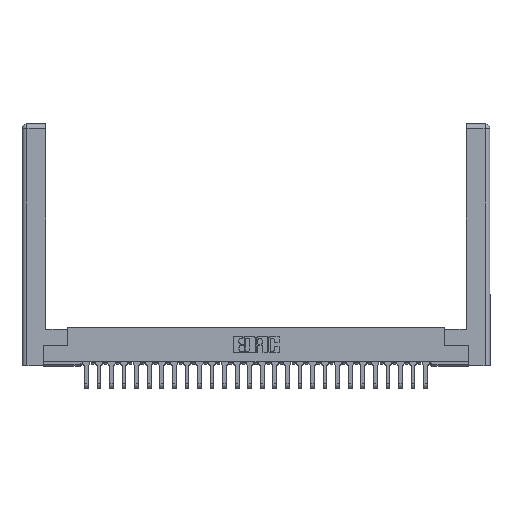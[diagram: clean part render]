
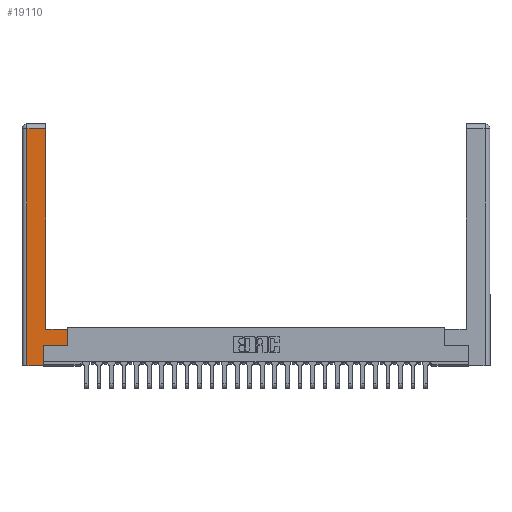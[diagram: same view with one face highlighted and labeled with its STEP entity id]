
A CAD part, top view. The second image highlights one B-rep face of the part: STEP entity #19110.
In plain terms, the highlighted planar face has unit normal (0, 0, 1).
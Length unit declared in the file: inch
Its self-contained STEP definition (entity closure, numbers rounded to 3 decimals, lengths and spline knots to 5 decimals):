
#45 = VECTOR ( 'NONE', #21171, 39.37008 ) ;
#301 = ORIENTED_EDGE ( 'NONE', *, *, #15538, .T. ) ;
#724 = VECTOR ( 'NONE', #25963, 39.37008 ) ;
#1144 = DIRECTION ( 'NONE',  ( 0., 1., 0. ) ) ;
#1430 = LINE ( 'NONE', #19168, #45 ) ;
#1854 = CARTESIAN_POINT ( 'NONE',  ( 0., 0., 0. ) ) ;
#1991 = EDGE_CURVE ( 'NONE', #27890, #3906, #9486, .T. ) ;
#2166 = CARTESIAN_POINT ( 'NONE',  ( 0.265, 0., 0. ) ) ;
#2806 = VECTOR ( 'NONE', #28010, 39.37008 ) ;
#3160 = LINE ( 'NONE', #28180, #6891 ) ;
#3191 = AXIS2_PLACEMENT_3D ( 'NONE', #1854, #6320, #17080 ) ;
#3430 = DIRECTION ( 'NONE',  ( 0., 1., 0. ) ) ;
#3699 = VERTEX_POINT ( 'NONE', #11754 ) ;
#3906 = VERTEX_POINT ( 'NONE', #21342 ) ;
#5853 = EDGE_CURVE ( 'NONE', #8416, #27890, #3160, .T. ) ;
#6320 = DIRECTION ( 'NONE',  ( 0., 0., -1. ) ) ;
#6891 = VECTOR ( 'NONE', #8741, 39.37008 ) ;
#7003 = CARTESIAN_POINT ( 'NONE',  ( 0.565, 0.245, 0. ) ) ;
#7031 = LINE ( 'NONE', #20258, #10799 ) ;
#7234 = LINE ( 'NONE', #2166, #724 ) ;
#7561 = CARTESIAN_POINT ( 'NONE',  ( 0.565, 0.45, 0. ) ) ;
#7753 = VERTEX_POINT ( 'NONE', #27652 ) ;
#8209 = CARTESIAN_POINT ( 'NONE',  ( 0.0615, 0., 0. ) ) ;
#8416 = VERTEX_POINT ( 'NONE', #11849 ) ;
#8741 = DIRECTION ( 'NONE',  ( 1., 0., 0. ) ) ;
#9172 = CARTESIAN_POINT ( 'NONE',  ( 0.0615, 2.94, 0. ) ) ;
#9486 = LINE ( 'NONE', #7561, #22222 ) ;
#9490 = VERTEX_POINT ( 'NONE', #9172 ) ;
#9682 = ORIENTED_EDGE ( 'NONE', *, *, #1991, .T. ) ;
#9726 = EDGE_CURVE ( 'NONE', #28029, #8416, #26314, .T. ) ;
#10799 = VECTOR ( 'NONE', #27554, 39.37008 ) ;
#11071 = FACE_OUTER_BOUND ( 'NONE', #18675, .T. ) ;
#11507 = ORIENTED_EDGE ( 'NONE', *, *, #5853, .T. ) ;
#11701 = VERTEX_POINT ( 'NONE', #20073 ) ;
#11754 = CARTESIAN_POINT ( 'NONE',  ( 0.295, 2.94, 0. ) ) ;
#11849 = CARTESIAN_POINT ( 'NONE',  ( 0.265, 0.245, 0. ) ) ;
#12340 = ORIENTED_EDGE ( 'NONE', *, *, #21503, .T. ) ;
#12440 = ORIENTED_EDGE ( 'NONE', *, *, #17039, .T. ) ;
#13300 = LINE ( 'NONE', #17403, #28079 ) ;
#14851 = ORIENTED_EDGE ( 'NONE', *, *, #9726, .T. ) ;
#14953 = VECTOR ( 'NONE', #3430, 39.37008 ) ;
#15538 = EDGE_CURVE ( 'NONE', #3699, #9490, #13300, .T. ) ;
#16528 = ORIENTED_EDGE ( 'NONE', *, *, #19633, .T. ) ;
#17039 = EDGE_CURVE ( 'NONE', #3906, #11701, #7031, .T. ) ;
#17080 = DIRECTION ( 'NONE',  ( -1., 0., 0. ) ) ;
#17403 = CARTESIAN_POINT ( 'NONE',  ( 0.0615, 2.94, 0. ) ) ;
#18675 = EDGE_LOOP ( 'NONE', ( #19070, #301, #16528, #12340, #14851, #11507, #9682, #12440 ) ) ;
#19070 = ORIENTED_EDGE ( 'NONE', *, *, #19674, .T. ) ;
#19110 = ADVANCED_FACE ( 'NONE', ( #11071 ), #19682, .F. ) ;
#19168 = CARTESIAN_POINT ( 'NONE',  ( 0.295, 3., 0. ) ) ;
#19633 = EDGE_CURVE ( 'NONE', #9490, #7753, #22014, .T. ) ;
#19674 = EDGE_CURVE ( 'NONE', #11701, #3699, #1430, .T. ) ;
#19682 = PLANE ( 'NONE',  #3191 ) ;
#20073 = CARTESIAN_POINT ( 'NONE',  ( 0.295, 0.45, 0. ) ) ;
#20258 = CARTESIAN_POINT ( 'NONE',  ( 0.295, 0.45, 0. ) ) ;
#21171 = DIRECTION ( 'NONE',  ( 0., 1., 0. ) ) ;
#21342 = CARTESIAN_POINT ( 'NONE',  ( 0.565, 0.45, 0. ) ) ;
#21503 = EDGE_CURVE ( 'NONE', #7753, #28029, #7234, .T. ) ;
#22014 = LINE ( 'NONE', #8209, #2806 ) ;
#22222 = VECTOR ( 'NONE', #1144, 39.37008 ) ;
#22835 = CARTESIAN_POINT ( 'NONE',  ( 0.265, 0., 0. ) ) ;
#23647 = DIRECTION ( 'NONE',  ( -1., 0., 0. ) ) ;
#25963 = DIRECTION ( 'NONE',  ( 1., 0., 0. ) ) ;
#26314 = LINE ( 'NONE', #27140, #14953 ) ;
#27140 = CARTESIAN_POINT ( 'NONE',  ( 0.265, 0.245, 0. ) ) ;
#27554 = DIRECTION ( 'NONE',  ( -1., 0., 0. ) ) ;
#27652 = CARTESIAN_POINT ( 'NONE',  ( 0.0615, 0., 0. ) ) ;
#27890 = VERTEX_POINT ( 'NONE', #7003 ) ;
#28010 = DIRECTION ( 'NONE',  ( 0., -1., 0. ) ) ;
#28029 = VERTEX_POINT ( 'NONE', #22835 ) ;
#28079 = VECTOR ( 'NONE', #23647, 39.37008 ) ;
#28180 = CARTESIAN_POINT ( 'NONE',  ( 0.565, 0.245, 0. ) ) ;
